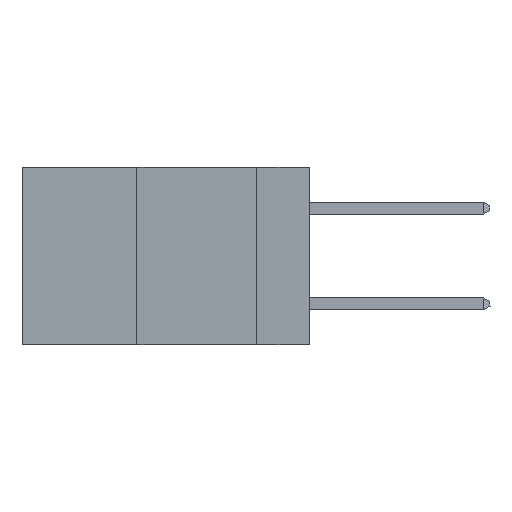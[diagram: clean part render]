
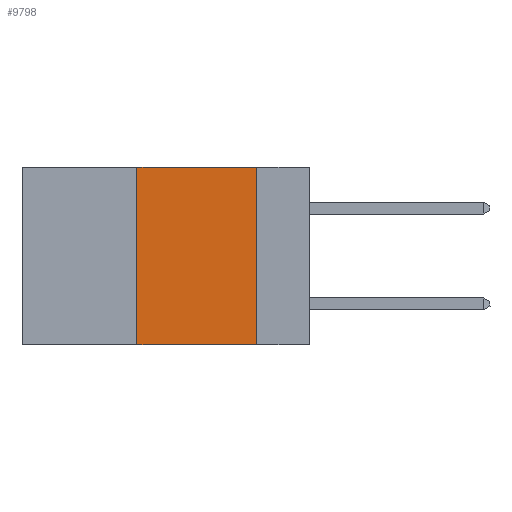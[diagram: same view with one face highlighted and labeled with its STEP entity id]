
A CAD part, left-side view. The second image highlights one B-rep face of the part: STEP entity #9798.
In plain terms, the highlighted planar face has unit normal (-1, 0, 0).
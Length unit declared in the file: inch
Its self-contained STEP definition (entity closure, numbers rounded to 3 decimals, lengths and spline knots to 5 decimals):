
#537 = PLANE ( 'NONE',  #1786 ) ;
#1325 = EDGE_CURVE ( 'NONE', #4793, #4398, #4312, .T. ) ;
#1403 = LINE ( 'NONE', #5120, #4029 ) ;
#1558 = DIRECTION ( 'NONE',  ( 1., 0., 0. ) ) ;
#1786 = AXIS2_PLACEMENT_3D ( 'NONE', #10098, #1558, #8379 ) ;
#2206 = LINE ( 'NONE', #9573, #9506 ) ;
#2864 = CARTESIAN_POINT ( 'NONE',  ( 0., 0.11, 0. ) ) ;
#4029 = VECTOR ( 'NONE', #7994, 39.37008 ) ;
#4312 = LINE ( 'NONE', #2864, #6920 ) ;
#4337 = CARTESIAN_POINT ( 'NONE',  ( 0., 0.6, -0.37 ) ) ;
#4398 = VERTEX_POINT ( 'NONE', #5801 ) ;
#4738 = ORIENTED_EDGE ( 'NONE', *, *, #7864, .F. ) ;
#4793 = VERTEX_POINT ( 'NONE', #11003 ) ;
#5120 = CARTESIAN_POINT ( 'NONE',  ( 0., 0.36, 0. ) ) ;
#5270 = EDGE_CURVE ( 'NONE', #10188, #4398, #12042, .T. ) ;
#5801 = CARTESIAN_POINT ( 'NONE',  ( 0., 0.11, -0.37 ) ) ;
#6030 = EDGE_LOOP ( 'NONE', ( #6479, #8148, #4738, #8557 ) ) ;
#6039 = CARTESIAN_POINT ( 'NONE',  ( 0., 0.36, -0.37 ) ) ;
#6316 = EDGE_CURVE ( 'NONE', #10839, #4793, #2206, .T. ) ;
#6479 = ORIENTED_EDGE ( 'NONE', *, *, #1325, .F. ) ;
#6770 = FACE_OUTER_BOUND ( 'NONE', #6030, .T. ) ;
#6920 = VECTOR ( 'NONE', #12157, 39.37008 ) ;
#6999 = VECTOR ( 'NONE', #11739, 39.37008 ) ;
#7864 = EDGE_CURVE ( 'NONE', #10188, #10839, #1403, .T. ) ;
#7994 = DIRECTION ( 'NONE',  ( 0., 0., 1. ) ) ;
#8148 = ORIENTED_EDGE ( 'NONE', *, *, #6316, .F. ) ;
#8379 = DIRECTION ( 'NONE',  ( 0., 0., -1. ) ) ;
#8557 = ORIENTED_EDGE ( 'NONE', *, *, #5270, .T. ) ;
#9506 = VECTOR ( 'NONE', #10418, 39.37008 ) ;
#9573 = CARTESIAN_POINT ( 'NONE',  ( 0., 0.6, 0. ) ) ;
#9798 = ADVANCED_FACE ( 'NONE', ( #6770 ), #537, .F. ) ;
#10098 = CARTESIAN_POINT ( 'NONE',  ( 0., 0.6, 0. ) ) ;
#10188 = VERTEX_POINT ( 'NONE', #6039 ) ;
#10418 = DIRECTION ( 'NONE',  ( 0., -1., 0. ) ) ;
#10839 = VERTEX_POINT ( 'NONE', #12296 ) ;
#11003 = CARTESIAN_POINT ( 'NONE',  ( 0., 0.11, 0. ) ) ;
#11739 = DIRECTION ( 'NONE',  ( 0., -1., 0. ) ) ;
#12042 = LINE ( 'NONE', #4337, #6999 ) ;
#12157 = DIRECTION ( 'NONE',  ( 0., 0., -1. ) ) ;
#12296 = CARTESIAN_POINT ( 'NONE',  ( 0., 0.36, 0. ) ) ;
